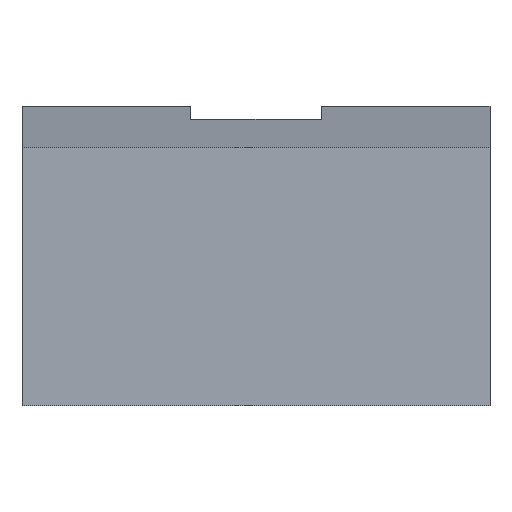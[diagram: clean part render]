
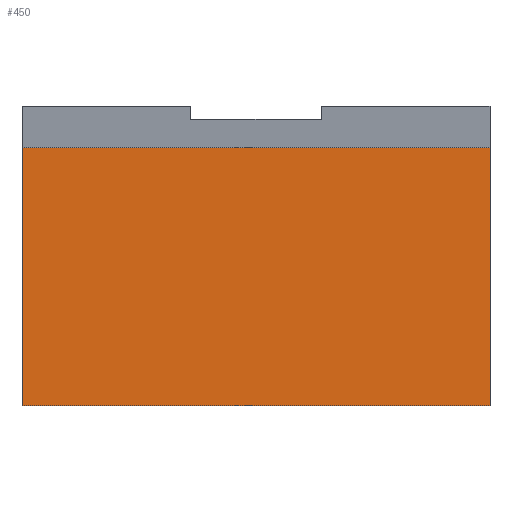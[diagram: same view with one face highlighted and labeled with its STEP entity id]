
A CAD part, front view. The second image highlights one B-rep face of the part: STEP entity #450.
In plain terms, the highlighted planar face has unit normal (0, -1, 0).
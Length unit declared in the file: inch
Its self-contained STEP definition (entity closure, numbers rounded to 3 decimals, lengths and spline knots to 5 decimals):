
#9 = LINE ( 'NONE', #132, #511 ) ;
#45 = ORIENTED_EDGE ( 'NONE', *, *, #597, .F. ) ;
#61 = CARTESIAN_POINT ( 'NONE',  ( 0.449, -2.534, 0. ) ) ;
#65 = DIRECTION ( 'NONE',  ( 0., 0., 1. ) ) ;
#122 = CARTESIAN_POINT ( 'NONE',  ( 0.449, -2.534, 0.49565 ) ) ;
#132 = CARTESIAN_POINT ( 'NONE',  ( 0.449, -2.534, 0. ) ) ;
#142 = CARTESIAN_POINT ( 'NONE',  ( -0.449, -2.534, 0. ) ) ;
#143 = DIRECTION ( 'NONE',  ( 0., -1., 0. ) ) ;
#166 = VERTEX_POINT ( 'NONE', #588 ) ;
#209 = LINE ( 'NONE', #469, #754 ) ;
#238 = ORIENTED_EDGE ( 'NONE', *, *, #333, .T. ) ;
#263 = VERTEX_POINT ( 'NONE', #122 ) ;
#285 = VECTOR ( 'NONE', #718, 39.37008 ) ;
#306 = VERTEX_POINT ( 'NONE', #61 ) ;
#333 = EDGE_CURVE ( 'NONE', #306, #263, #9, .T. ) ;
#408 = ORIENTED_EDGE ( 'NONE', *, *, #425, .F. ) ;
#425 = EDGE_CURVE ( 'NONE', #515, #166, #559, .T. ) ;
#438 = CARTESIAN_POINT ( 'NONE',  ( -0.449, -2.534, 0. ) ) ;
#450 = ADVANCED_FACE ( 'NONE', ( #536 ), #644, .T. ) ;
#469 = CARTESIAN_POINT ( 'NONE',  ( 0.449, -2.534, 0. ) ) ;
#511 = VECTOR ( 'NONE', #65, 39.37008 ) ;
#513 = EDGE_CURVE ( 'NONE', #263, #166, #839, .T. ) ;
#515 = VERTEX_POINT ( 'NONE', #438 ) ;
#536 = FACE_OUTER_BOUND ( 'NONE', #818, .T. ) ;
#559 = LINE ( 'NONE', #142, #725 ) ;
#569 = CARTESIAN_POINT ( 'NONE',  ( 0.449, -2.534, 0. ) ) ;
#582 = AXIS2_PLACEMENT_3D ( 'NONE', #569, #143, #646 ) ;
#588 = CARTESIAN_POINT ( 'NONE',  ( -0.449, -2.534, 0.49565 ) ) ;
#597 = EDGE_CURVE ( 'NONE', #306, #515, #209, .T. ) ;
#644 = PLANE ( 'NONE',  #582 ) ;
#646 = DIRECTION ( 'NONE',  ( 0., 0., -1. ) ) ;
#652 = CARTESIAN_POINT ( 'NONE',  ( 0.449, -2.534, 0.49565 ) ) ;
#718 = DIRECTION ( 'NONE',  ( -1., 0., 0. ) ) ;
#725 = VECTOR ( 'NONE', #776, 39.37008 ) ;
#744 = DIRECTION ( 'NONE',  ( -1., 0., 0. ) ) ;
#754 = VECTOR ( 'NONE', #744, 39.37008 ) ;
#769 = ORIENTED_EDGE ( 'NONE', *, *, #513, .T. ) ;
#776 = DIRECTION ( 'NONE',  ( 0., 0., 1. ) ) ;
#818 = EDGE_LOOP ( 'NONE', ( #408, #45, #238, #769 ) ) ;
#839 = LINE ( 'NONE', #652, #285 ) ;
